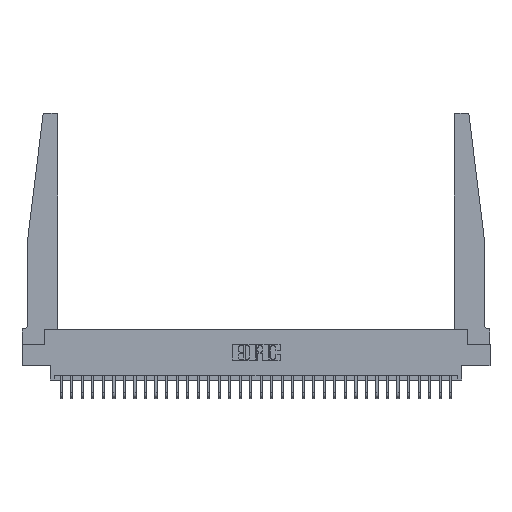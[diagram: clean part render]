
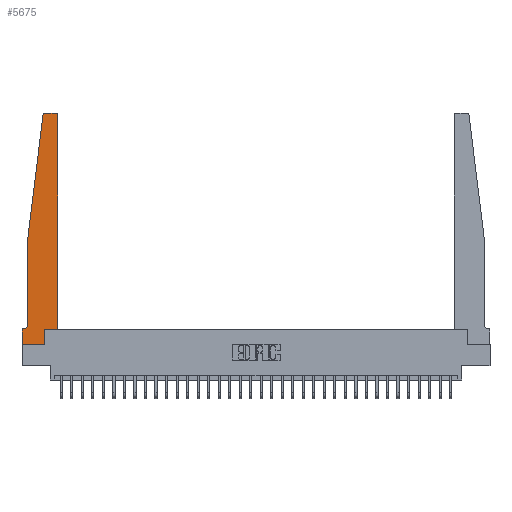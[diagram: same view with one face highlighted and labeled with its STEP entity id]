
A CAD part, top view. The second image highlights one B-rep face of the part: STEP entity #5675.
In plain terms, the highlighted planar face has unit normal (0, 0, 1).
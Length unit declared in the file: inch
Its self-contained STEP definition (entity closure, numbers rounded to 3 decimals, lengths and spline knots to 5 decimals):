
#181 = CARTESIAN_POINT ( 'NONE',  ( 0.065, 0.1875, 0.37 ) ) ;
#964 = CARTESIAN_POINT ( 'NONE',  ( 0.425, 0.18, 0.37 ) ) ;
#1326 = ORIENTED_EDGE ( 'NONE', *, *, #5013, .T. ) ;
#1410 = CARTESIAN_POINT ( 'NONE',  ( 0.065, 1.25, 0.37 ) ) ;
#1502 = EDGE_CURVE ( 'NONE', #10064, #10764, #18098, .T. ) ;
#1599 = DIRECTION ( 'NONE',  ( 0., 1., 0. ) ) ;
#1624 = EDGE_LOOP ( 'NONE', ( #22541, #15079, #6866, #13403, #28422, #25773, #10296, #26857, #1326, #12986, #24189, #19042 ) ) ;
#2062 = CARTESIAN_POINT ( 'NONE',  ( 0.27653, 2.75, 0.37 ) ) ;
#2102 = AXIS2_PLACEMENT_3D ( 'NONE', #10227, #19605, #7583 ) ;
#2255 = CARTESIAN_POINT ( 'NONE',  ( 0.25, 2.75, 0.37 ) ) ;
#2938 = LINE ( 'NONE', #964, #12918 ) ;
#3462 = EDGE_CURVE ( 'NONE', #19137, #29658, #24615, .T. ) ;
#3695 = VECTOR ( 'NONE', #22946, 39.37008 ) ;
#4176 = CIRCLE ( 'NONE', #2102, 0.03 ) ;
#4655 = VECTOR ( 'NONE', #27479, 39.37008 ) ;
#4700 = LINE ( 'NONE', #7157, #21551 ) ;
#4757 = CIRCLE ( 'NONE', #26299, 0.05 ) ;
#4973 = CARTESIAN_POINT ( 'NONE',  ( 0.2605, 0.18, 0.37 ) ) ;
#5013 = EDGE_CURVE ( 'NONE', #21650, #17887, #12024, .T. ) ;
#5675 = ADVANCED_FACE ( 'NONE', ( #22111 ), #26880, .T. ) ;
#5738 = EDGE_CURVE ( 'NONE', #27264, #10064, #4757, .T. ) ;
#6733 = EDGE_CURVE ( 'NONE', #17887, #17527, #2938, .T. ) ;
#6801 = DIRECTION ( 'NONE',  ( 1., 0., 0. ) ) ;
#6866 = ORIENTED_EDGE ( 'NONE', *, *, #28706, .T. ) ;
#7157 = CARTESIAN_POINT ( 'NONE',  ( 0.425, 0.18, 0.37 ) ) ;
#7583 = DIRECTION ( 'NONE',  ( 1., 0., 0. ) ) ;
#7626 = CARTESIAN_POINT ( 'NONE',  ( 0.065, 1.25, 0.37 ) ) ;
#8058 = CARTESIAN_POINT ( 'NONE',  ( 0., 0., 0.37 ) ) ;
#8227 = AXIS2_PLACEMENT_3D ( 'NONE', #13677, #28011, #18472 ) ;
#9765 = CARTESIAN_POINT ( 'NONE',  ( 0.395, 2.75, 0.37 ) ) ;
#9928 = VERTEX_POINT ( 'NONE', #23538 ) ;
#9950 = CARTESIAN_POINT ( 'NONE',  ( 0.425, 0.18, 0.37 ) ) ;
#10064 = VERTEX_POINT ( 'NONE', #29293 ) ;
#10227 = CARTESIAN_POINT ( 'NONE',  ( 0.395, 2.72, 0.37 ) ) ;
#10296 = ORIENTED_EDGE ( 'NONE', *, *, #12372, .T. ) ;
#10528 = DIRECTION ( 'NONE',  ( -0.122, -0.992, 0. ) ) ;
#10764 = VERTEX_POINT ( 'NONE', #10811 ) ;
#10811 = CARTESIAN_POINT ( 'NONE',  ( 0., 0.1875, 0.37 ) ) ;
#10970 = LINE ( 'NONE', #27033, #12296 ) ;
#12024 = LINE ( 'NONE', #29639, #4655 ) ;
#12192 = EDGE_CURVE ( 'NONE', #17527, #17500, #4700, .T. ) ;
#12296 = VECTOR ( 'NONE', #26101, 39.37008 ) ;
#12372 = EDGE_CURVE ( 'NONE', #10764, #21910, #30200, .T. ) ;
#12412 = CARTESIAN_POINT ( 'NONE',  ( 0.425, 2.72, 0.37 ) ) ;
#12918 = VECTOR ( 'NONE', #20519, 39.37008 ) ;
#12986 = ORIENTED_EDGE ( 'NONE', *, *, #6733, .T. ) ;
#13143 = EDGE_CURVE ( 'NONE', #17500, #19137, #4176, .T. ) ;
#13403 = ORIENTED_EDGE ( 'NONE', *, *, #24262, .T. ) ;
#13677 = CARTESIAN_POINT ( 'NONE',  ( 0.27653, 2.72, 0.37 ) ) ;
#13883 = LINE ( 'NONE', #1410, #18241 ) ;
#14039 = DIRECTION ( 'NONE',  ( 0., 0., -1. ) ) ;
#14482 = CARTESIAN_POINT ( 'NONE',  ( 0.065, 0.2375, 0.37 ) ) ;
#14888 = CARTESIAN_POINT ( 'NONE',  ( 0., 0., 0.37 ) ) ;
#15079 = ORIENTED_EDGE ( 'NONE', *, *, #23349, .T. ) ;
#16359 = DIRECTION ( 'NONE',  ( 0., -1., 0. ) ) ;
#17009 = CARTESIAN_POINT ( 'NONE',  ( 0., 0.1875, 0.37 ) ) ;
#17500 = VERTEX_POINT ( 'NONE', #12412 ) ;
#17527 = VERTEX_POINT ( 'NONE', #9950 ) ;
#17887 = VERTEX_POINT ( 'NONE', #4973 ) ;
#18098 = LINE ( 'NONE', #181, #27962 ) ;
#18241 = VECTOR ( 'NONE', #16359, 39.37008 ) ;
#18472 = DIRECTION ( 'NONE',  ( 1., 0., 0. ) ) ;
#19042 = ORIENTED_EDGE ( 'NONE', *, *, #13143, .T. ) ;
#19052 = EDGE_CURVE ( 'NONE', #21910, #21650, #10970, .T. ) ;
#19062 = VECTOR ( 'NONE', #10528, 39.37008 ) ;
#19137 = VERTEX_POINT ( 'NONE', #9765 ) ;
#19605 = DIRECTION ( 'NONE',  ( 0., 0., 1. ) ) ;
#20519 = DIRECTION ( 'NONE',  ( 1., 0., 0. ) ) ;
#21551 = VECTOR ( 'NONE', #1599, 39.37008 ) ;
#21650 = VERTEX_POINT ( 'NONE', #22230 ) ;
#21910 = VERTEX_POINT ( 'NONE', #8058 ) ;
#22111 = FACE_OUTER_BOUND ( 'NONE', #1624, .T. ) ;
#22230 = CARTESIAN_POINT ( 'NONE',  ( 0.2605, 0., 0.37 ) ) ;
#22541 = ORIENTED_EDGE ( 'NONE', *, *, #3462, .T. ) ;
#22546 = CARTESIAN_POINT ( 'NONE',  ( 0.065, 1.25, 0.37 ) ) ;
#22611 = AXIS2_PLACEMENT_3D ( 'NONE', #17009, #32143, #6801 ) ;
#22946 = DIRECTION ( 'NONE',  ( 0., -1., 0. ) ) ;
#23349 = EDGE_CURVE ( 'NONE', #29658, #9928, #31885, .T. ) ;
#23538 = CARTESIAN_POINT ( 'NONE',  ( 0.24675, 2.72367, 0.37 ) ) ;
#24189 = ORIENTED_EDGE ( 'NONE', *, *, #12192, .T. ) ;
#24262 = EDGE_CURVE ( 'NONE', #29713, #27264, #13883, .T. ) ;
#24615 = LINE ( 'NONE', #2255, #25313 ) ;
#25168 = LINE ( 'NONE', #22546, #19062 ) ;
#25313 = VECTOR ( 'NONE', #32017, 39.37008 ) ;
#25773 = ORIENTED_EDGE ( 'NONE', *, *, #1502, .T. ) ;
#26101 = DIRECTION ( 'NONE',  ( 1., 0., 0. ) ) ;
#26299 = AXIS2_PLACEMENT_3D ( 'NONE', #26552, #14039, #31981 ) ;
#26552 = CARTESIAN_POINT ( 'NONE',  ( 0.015, 0.2375, 0.37 ) ) ;
#26857 = ORIENTED_EDGE ( 'NONE', *, *, #19052, .T. ) ;
#26880 = PLANE ( 'NONE',  #22611 ) ;
#27033 = CARTESIAN_POINT ( 'NONE',  ( 0., 0., 0.37 ) ) ;
#27264 = VERTEX_POINT ( 'NONE', #14482 ) ;
#27479 = DIRECTION ( 'NONE',  ( 0., 1., 0. ) ) ;
#27962 = VECTOR ( 'NONE', #28121, 39.37008 ) ;
#28011 = DIRECTION ( 'NONE',  ( 0., 0., 1. ) ) ;
#28121 = DIRECTION ( 'NONE',  ( -1., 0., 0. ) ) ;
#28422 = ORIENTED_EDGE ( 'NONE', *, *, #5738, .T. ) ;
#28706 = EDGE_CURVE ( 'NONE', #9928, #29713, #25168, .T. ) ;
#29293 = CARTESIAN_POINT ( 'NONE',  ( 0.015, 0.1875, 0.37 ) ) ;
#29639 = CARTESIAN_POINT ( 'NONE',  ( 0.2605, 0.18, 0.37 ) ) ;
#29658 = VERTEX_POINT ( 'NONE', #2062 ) ;
#29713 = VERTEX_POINT ( 'NONE', #7626 ) ;
#30200 = LINE ( 'NONE', #14888, #3695 ) ;
#31885 = CIRCLE ( 'NONE', #8227, 0.03 ) ;
#31981 = DIRECTION ( 'NONE',  ( -1., 0., 0. ) ) ;
#32017 = DIRECTION ( 'NONE',  ( -1., 0., 0. ) ) ;
#32143 = DIRECTION ( 'NONE',  ( 0., 0., 1. ) ) ;
